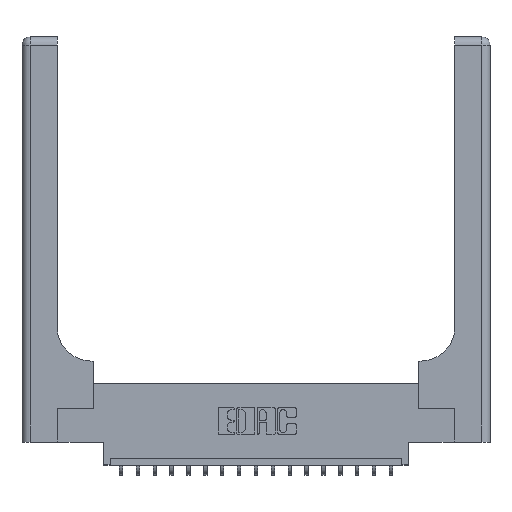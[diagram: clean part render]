
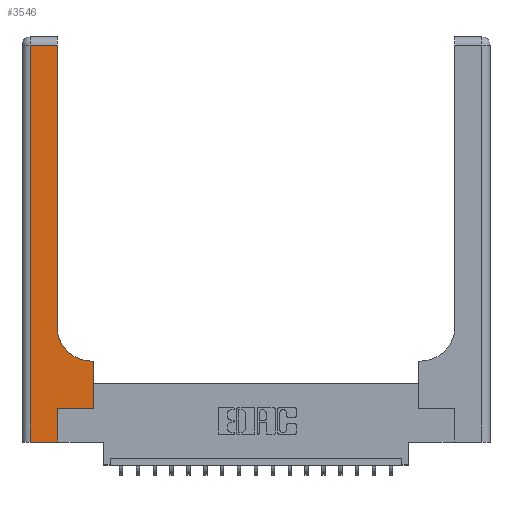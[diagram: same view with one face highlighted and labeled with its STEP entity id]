
A CAD part, top view. The second image highlights one B-rep face of the part: STEP entity #3546.
In plain terms, the highlighted planar face has unit normal (0, 0, 1).
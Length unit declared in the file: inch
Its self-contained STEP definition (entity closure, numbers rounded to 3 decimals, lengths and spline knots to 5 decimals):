
#137 = LINE ( 'NONE', #4901, #3898 ) ;
#346 = VERTEX_POINT ( 'NONE', #1804 ) ;
#471 = VERTEX_POINT ( 'NONE', #9895 ) ;
#911 = ORIENTED_EDGE ( 'NONE', *, *, #1223, .T. ) ;
#1223 = EDGE_CURVE ( 'NONE', #3465, #8583, #137, .T. ) ;
#1605 = DIRECTION ( 'NONE',  ( 1., 0., 0. ) ) ;
#1804 = CARTESIAN_POINT ( 'NONE',  ( 0.265, 0., 0.37 ) ) ;
#1884 = VECTOR ( 'NONE', #7544, 39.37008 ) ;
#1959 = DIRECTION ( 'NONE',  ( 0., 0., -1. ) ) ;
#2709 = PLANE ( 'NONE',  #16287 ) ;
#2743 = ORIENTED_EDGE ( 'NONE', *, *, #8061, .T. ) ;
#3307 = CARTESIAN_POINT ( 'NONE',  ( 0.26, 0.85, 0.37 ) ) ;
#3465 = VERTEX_POINT ( 'NONE', #8616 ) ;
#3504 = CARTESIAN_POINT ( 'NONE',  ( 0.265, 0., 0.37 ) ) ;
#3546 = ADVANCED_FACE ( 'NONE', ( #18322 ), #2709, .F. ) ;
#3883 = EDGE_CURVE ( 'NONE', #10649, #19230, #15661, .T. ) ;
#3898 = VECTOR ( 'NONE', #12311, 39.37008 ) ;
#3923 = LINE ( 'NONE', #7032, #16431 ) ;
#4305 = DIRECTION ( 'NONE',  ( -1., 0., 0. ) ) ;
#4424 = LINE ( 'NONE', #18550, #1884 ) ;
#4600 = LINE ( 'NONE', #9207, #8332 ) ;
#4617 = VECTOR ( 'NONE', #11079, 39.37008 ) ;
#4815 = ORIENTED_EDGE ( 'NONE', *, *, #3883, .T. ) ;
#4901 = CARTESIAN_POINT ( 'NONE',  ( 0.06, 3., 0.37 ) ) ;
#4912 = EDGE_CURVE ( 'NONE', #346, #471, #17030, .T. ) ;
#5523 = DIRECTION ( 'NONE',  ( 0., 1., 0. ) ) ;
#5736 = VERTEX_POINT ( 'NONE', #6851 ) ;
#5954 = LINE ( 'NONE', #19581, #12233 ) ;
#6243 = CARTESIAN_POINT ( 'NONE',  ( 0.26, 3., 0.37 ) ) ;
#6596 = CARTESIAN_POINT ( 'NONE',  ( 0.528, 0.6, 0.37 ) ) ;
#6851 = CARTESIAN_POINT ( 'NONE',  ( 0.51, 0.6, 0.37 ) ) ;
#6976 = CARTESIAN_POINT ( 'NONE',  ( 0.06, 0., 0.37 ) ) ;
#7032 = CARTESIAN_POINT ( 'NONE',  ( 0.528, 0.25, 0.37 ) ) ;
#7067 = EDGE_CURVE ( 'NONE', #5736, #10649, #11697, .T. ) ;
#7323 = CARTESIAN_POINT ( 'NONE',  ( 0.26, 2.94, 0.37 ) ) ;
#7544 = DIRECTION ( 'NONE',  ( 1., 0., 0. ) ) ;
#7858 = AXIS2_PLACEMENT_3D ( 'NONE', #10042, #1959, #8069 ) ;
#8061 = EDGE_CURVE ( 'NONE', #19107, #10756, #3923, .T. ) ;
#8069 = DIRECTION ( 'NONE',  ( 1., 0., 0. ) ) ;
#8207 = LINE ( 'NONE', #17307, #4617 ) ;
#8218 = ORIENTED_EDGE ( 'NONE', *, *, #4912, .T. ) ;
#8320 = VECTOR ( 'NONE', #9356, 39.37008 ) ;
#8332 = VECTOR ( 'NONE', #1605, 39.37008 ) ;
#8480 = ORIENTED_EDGE ( 'NONE', *, *, #9498, .T. ) ;
#8583 = VERTEX_POINT ( 'NONE', #6976 ) ;
#8616 = CARTESIAN_POINT ( 'NONE',  ( 0.06, 2.94, 0.37 ) ) ;
#8854 = ORIENTED_EDGE ( 'NONE', *, *, #7067, .T. ) ;
#9207 = CARTESIAN_POINT ( 'NONE',  ( 0.265, 0.25, 0.37 ) ) ;
#9356 = DIRECTION ( 'NONE',  ( 0., 1., 0. ) ) ;
#9421 = DIRECTION ( 'NONE',  ( 0., 1., 0. ) ) ;
#9498 = EDGE_CURVE ( 'NONE', #471, #19107, #4600, .T. ) ;
#9895 = CARTESIAN_POINT ( 'NONE',  ( 0.265, 0.25, 0.37 ) ) ;
#10040 = EDGE_LOOP ( 'NONE', ( #4815, #18670, #911, #13278, #8218, #8480, #2743, #11905, #8854 ) ) ;
#10042 = CARTESIAN_POINT ( 'NONE',  ( 0.51, 0.85, 0.37 ) ) ;
#10649 = VERTEX_POINT ( 'NONE', #3307 ) ;
#10756 = VERTEX_POINT ( 'NONE', #6596 ) ;
#11079 = DIRECTION ( 'NONE',  ( -1., 0., 0. ) ) ;
#11697 = CIRCLE ( 'NONE', #7858, 0.25 ) ;
#11718 = EDGE_CURVE ( 'NONE', #8583, #346, #4424, .T. ) ;
#11905 = ORIENTED_EDGE ( 'NONE', *, *, #13920, .T. ) ;
#11913 = CARTESIAN_POINT ( 'NONE',  ( 0., 3., 0.37 ) ) ;
#12064 = DIRECTION ( 'NONE',  ( -1., 0., 0. ) ) ;
#12233 = VECTOR ( 'NONE', #12064, 39.37008 ) ;
#12311 = DIRECTION ( 'NONE',  ( 0., -1., 0. ) ) ;
#12528 = VECTOR ( 'NONE', #9421, 39.37008 ) ;
#13278 = ORIENTED_EDGE ( 'NONE', *, *, #11718, .T. ) ;
#13920 = EDGE_CURVE ( 'NONE', #10756, #5736, #8207, .T. ) ;
#15661 = LINE ( 'NONE', #6243, #8320 ) ;
#16048 = CARTESIAN_POINT ( 'NONE',  ( 0.528, 0.25, 0.37 ) ) ;
#16287 = AXIS2_PLACEMENT_3D ( 'NONE', #11913, #18023, #4305 ) ;
#16431 = VECTOR ( 'NONE', #5523, 39.37008 ) ;
#17030 = LINE ( 'NONE', #3504, #12528 ) ;
#17307 = CARTESIAN_POINT ( 'NONE',  ( 0.26, 0.6, 0.37 ) ) ;
#18023 = DIRECTION ( 'NONE',  ( 0., 0., -1. ) ) ;
#18322 = FACE_OUTER_BOUND ( 'NONE', #10040, .T. ) ;
#18495 = EDGE_CURVE ( 'NONE', #19230, #3465, #5954, .T. ) ;
#18550 = CARTESIAN_POINT ( 'NONE',  ( 0., 0., 0.37 ) ) ;
#18670 = ORIENTED_EDGE ( 'NONE', *, *, #18495, .T. ) ;
#19107 = VERTEX_POINT ( 'NONE', #16048 ) ;
#19230 = VERTEX_POINT ( 'NONE', #7323 ) ;
#19581 = CARTESIAN_POINT ( 'NONE',  ( 0., 2.94, 0.37 ) ) ;
